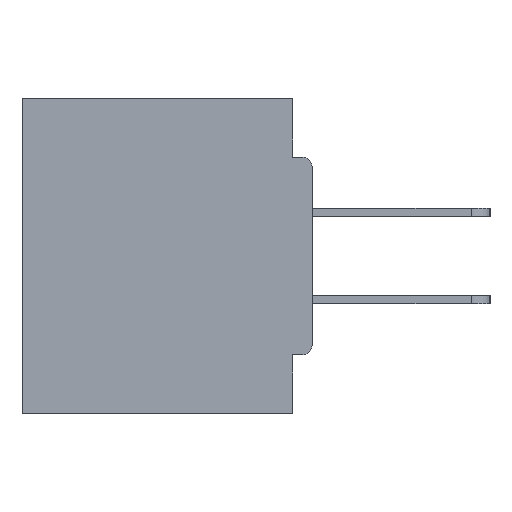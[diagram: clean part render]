
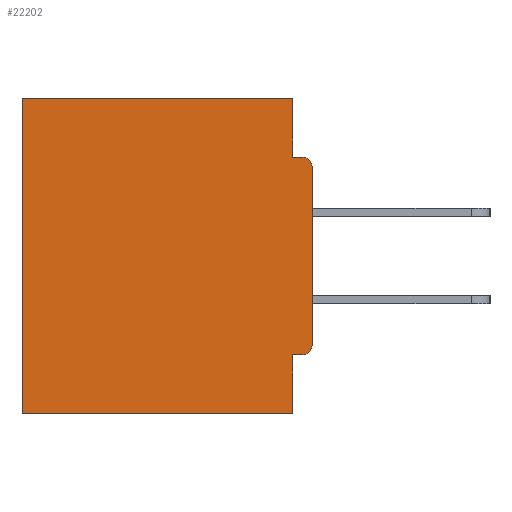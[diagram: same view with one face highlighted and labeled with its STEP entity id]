
A CAD part, left-side view. The second image highlights one B-rep face of the part: STEP entity #22202.
In plain terms, the highlighted planar face has unit normal (-1, 0, 0).
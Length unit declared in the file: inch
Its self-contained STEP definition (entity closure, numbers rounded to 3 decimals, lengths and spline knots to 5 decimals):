
#2296 = EDGE_CURVE ( 'NONE', #27808, #23096, #19927, .T. ) ;
#2678 = ORIENTED_EDGE ( 'NONE', *, *, #11149, .F. ) ;
#2780 = DIRECTION ( 'NONE',  ( 0., 0., -1. ) ) ;
#3166 = LINE ( 'NONE', #13531, #13972 ) ;
#3527 = DIRECTION ( 'NONE',  ( 0., 0., -1. ) ) ;
#3965 = FACE_OUTER_BOUND ( 'NONE', #12655, .T. ) ;
#4706 = DIRECTION ( 'NONE',  ( 0., 1., 0. ) ) ;
#4822 = CARTESIAN_POINT ( 'NONE',  ( 0.298, 0., 0. ) ) ;
#4860 = LINE ( 'NONE', #24320, #19478 ) ;
#4967 = ORIENTED_EDGE ( 'NONE', *, *, #6311, .F. ) ;
#5249 = AXIS2_PLACEMENT_3D ( 'NONE', #19712, #16965, #30290 ) ;
#5424 = ORIENTED_EDGE ( 'NONE', *, *, #10724, .T. ) ;
#6002 = EDGE_CURVE ( 'NONE', #17965, #22740, #4860, .T. ) ;
#6311 = EDGE_CURVE ( 'NONE', #22740, #20899, #25423, .T. ) ;
#6451 = EDGE_CURVE ( 'NONE', #23096, #20899, #8272, .T. ) ;
#7016 = ORIENTED_EDGE ( 'NONE', *, *, #6002, .F. ) ;
#7862 = AXIS2_PLACEMENT_3D ( 'NONE', #31951, #12668, #12903 ) ;
#7926 = ORIENTED_EDGE ( 'NONE', *, *, #32635, .F. ) ;
#8272 = LINE ( 'NONE', #13516, #27540 ) ;
#9303 = ORIENTED_EDGE ( 'NONE', *, *, #6451, .T. ) ;
#10557 = EDGE_CURVE ( 'NONE', #16153, #32423, #35060, .T. ) ;
#10724 = EDGE_CURVE ( 'NONE', #11358, #34397, #12318, .T. ) ;
#11149 = EDGE_CURVE ( 'NONE', #27808, #19693, #16542, .T. ) ;
#11220 = CARTESIAN_POINT ( 'NONE',  ( 0.298, 0.031, 0. ) ) ;
#11358 = VERTEX_POINT ( 'NONE', #25606 ) ;
#12318 = CIRCLE ( 'NONE', #5249, 0.015 ) ;
#12655 = EDGE_LOOP ( 'NONE', ( #18745, #7926, #2678, #26171, #9303, #4967, #7016, #21908, #5424, #19745 ) ) ;
#12668 = DIRECTION ( 'NONE',  ( 1., 0., 0. ) ) ;
#12903 = DIRECTION ( 'NONE',  ( 0., 0., -1. ) ) ;
#13030 = VECTOR ( 'NONE', #35230, 39.37008 ) ;
#13123 = CARTESIAN_POINT ( 'NONE',  ( 0.298, 0., -0.3915 ) ) ;
#13516 = CARTESIAN_POINT ( 'NONE',  ( 0.298, 0.46, 0. ) ) ;
#13531 = CARTESIAN_POINT ( 'NONE',  ( 0.298, 0., 0. ) ) ;
#13777 = VECTOR ( 'NONE', #15575, 39.37008 ) ;
#13944 = EDGE_CURVE ( 'NONE', #16153, #34397, #3166, .T. ) ;
#13972 = VECTOR ( 'NONE', #2780, 39.37008 ) ;
#15575 = DIRECTION ( 'NONE',  ( 0., -1., 0. ) ) ;
#16153 = VERTEX_POINT ( 'NONE', #34289 ) ;
#16235 = CARTESIAN_POINT ( 'NONE',  ( 0.298, 0.031, -0.4065 ) ) ;
#16542 = LINE ( 'NONE', #20895, #22532 ) ;
#16965 = DIRECTION ( 'NONE',  ( -1., 0., 0. ) ) ;
#17965 = VERTEX_POINT ( 'NONE', #16235 ) ;
#18202 = VECTOR ( 'NONE', #4706, 39.37008 ) ;
#18651 = DIRECTION ( 'NONE',  ( -1., 0., 0. ) ) ;
#18656 = CARTESIAN_POINT ( 'NONE',  ( 0.298, 0., -0.5 ) ) ;
#18745 = ORIENTED_EDGE ( 'NONE', *, *, #10557, .T. ) ;
#19478 = VECTOR ( 'NONE', #3527, 39.37008 ) ;
#19693 = VERTEX_POINT ( 'NONE', #32024 ) ;
#19712 = CARTESIAN_POINT ( 'NONE',  ( 0.298, 0.015, -0.3915 ) ) ;
#19745 = ORIENTED_EDGE ( 'NONE', *, *, #13944, .F. ) ;
#19815 = CARTESIAN_POINT ( 'NONE',  ( 0.298, 0.46, -0.5 ) ) ;
#19927 = LINE ( 'NONE', #4822, #18202 ) ;
#20320 = EDGE_CURVE ( 'NONE', #11358, #17965, #34170, .T. ) ;
#20895 = CARTESIAN_POINT ( 'NONE',  ( 0.298, 0.031, -0.5 ) ) ;
#20899 = VERTEX_POINT ( 'NONE', #19815 ) ;
#21041 = LINE ( 'NONE', #23794, #13777 ) ;
#21908 = ORIENTED_EDGE ( 'NONE', *, *, #20320, .F. ) ;
#22202 = ADVANCED_FACE ( 'NONE', ( #3965 ), #34730, .F. ) ;
#22532 = VECTOR ( 'NONE', #23733, 39.37008 ) ;
#22740 = VERTEX_POINT ( 'NONE', #23716 ) ;
#23096 = VERTEX_POINT ( 'NONE', #26076 ) ;
#23716 = CARTESIAN_POINT ( 'NONE',  ( 0.298, 0.031, -0.5 ) ) ;
#23733 = DIRECTION ( 'NONE',  ( 0., 0., -1. ) ) ;
#23794 = CARTESIAN_POINT ( 'NONE',  ( 0.298, 0., -0.0935 ) ) ;
#24320 = CARTESIAN_POINT ( 'NONE',  ( 0.298, 0.031, -0.5 ) ) ;
#25423 = LINE ( 'NONE', #18656, #13030 ) ;
#25606 = CARTESIAN_POINT ( 'NONE',  ( 0.298, 0.015, -0.4065 ) ) ;
#25639 = CARTESIAN_POINT ( 'NONE',  ( 0.298, 0.015, -0.0935 ) ) ;
#26076 = CARTESIAN_POINT ( 'NONE',  ( 0.298, 0.46, 0. ) ) ;
#26171 = ORIENTED_EDGE ( 'NONE', *, *, #2296, .T. ) ;
#26799 = VECTOR ( 'NONE', #29468, 39.37008 ) ;
#27314 = AXIS2_PLACEMENT_3D ( 'NONE', #35343, #18651, #35575 ) ;
#27540 = VECTOR ( 'NONE', #33060, 39.37008 ) ;
#27808 = VERTEX_POINT ( 'NONE', #11220 ) ;
#29468 = DIRECTION ( 'NONE',  ( 0., 1., 0. ) ) ;
#30290 = DIRECTION ( 'NONE',  ( 0., 0., -1. ) ) ;
#31951 = CARTESIAN_POINT ( 'NONE',  ( 0.298, 0., 0. ) ) ;
#32024 = CARTESIAN_POINT ( 'NONE',  ( 0.298, 0.031, -0.0935 ) ) ;
#32423 = VERTEX_POINT ( 'NONE', #25639 ) ;
#32635 = EDGE_CURVE ( 'NONE', #19693, #32423, #21041, .T. ) ;
#33060 = DIRECTION ( 'NONE',  ( 0., 0., -1. ) ) ;
#34170 = LINE ( 'NONE', #34644, #26799 ) ;
#34289 = CARTESIAN_POINT ( 'NONE',  ( 0.298, 0., -0.1085 ) ) ;
#34397 = VERTEX_POINT ( 'NONE', #13123 ) ;
#34644 = CARTESIAN_POINT ( 'NONE',  ( 0.298, 0., -0.4065 ) ) ;
#34730 = PLANE ( 'NONE',  #7862 ) ;
#35060 = CIRCLE ( 'NONE', #27314, 0.015 ) ;
#35230 = DIRECTION ( 'NONE',  ( 0., 1., 0. ) ) ;
#35343 = CARTESIAN_POINT ( 'NONE',  ( 0.298, 0.015, -0.1085 ) ) ;
#35575 = DIRECTION ( 'NONE',  ( 0., 0., -1. ) ) ;
